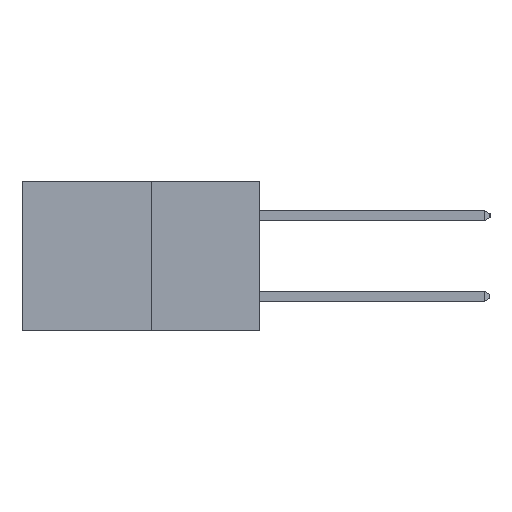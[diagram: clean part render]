
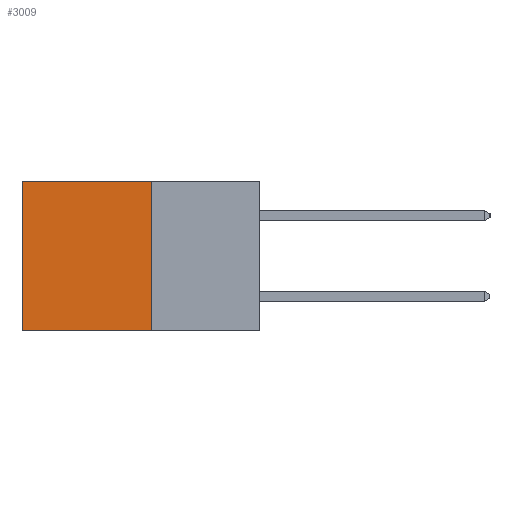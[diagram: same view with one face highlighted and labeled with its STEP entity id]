
A CAD part, left-side view. The second image highlights one B-rep face of the part: STEP entity #3009.
In plain terms, the highlighted planar face has unit normal (-1, 0, 0).
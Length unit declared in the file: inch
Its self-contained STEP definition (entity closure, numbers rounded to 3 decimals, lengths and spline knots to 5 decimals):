
#1442 = CARTESIAN_POINT ( 'NONE',  ( 0.277, 0.27, 0. ) ) ;
#1507 = DIRECTION ( 'NONE',  ( 0., 0., -1. ) ) ;
#1745 = CARTESIAN_POINT ( 'NONE',  ( 0.277, 0.59, -0.37 ) ) ;
#1864 = LINE ( 'NONE', #1745, #9454 ) ;
#1906 = ORIENTED_EDGE ( 'NONE', *, *, #1978, .F. ) ;
#1978 = EDGE_CURVE ( 'NONE', #2466, #4831, #8914, .T. ) ;
#2058 = AXIS2_PLACEMENT_3D ( 'NONE', #5462, #4256, #4336 ) ;
#2251 = EDGE_LOOP ( 'NONE', ( #9683, #1906, #9900, #2403 ) ) ;
#2360 = DIRECTION ( 'NONE',  ( 0., 1., 0. ) ) ;
#2403 = ORIENTED_EDGE ( 'NONE', *, *, #3739, .T. ) ;
#2466 = VERTEX_POINT ( 'NONE', #8448 ) ;
#3009 = ADVANCED_FACE ( 'NONE', ( #5293 ), #5412, .F. ) ;
#3052 = LINE ( 'NONE', #9658, #6705 ) ;
#3739 = EDGE_CURVE ( 'NONE', #8622, #4681, #6283, .T. ) ;
#4256 = DIRECTION ( 'NONE',  ( 1., 0., 0. ) ) ;
#4336 = DIRECTION ( 'NONE',  ( 0., 0., -1. ) ) ;
#4681 = VERTEX_POINT ( 'NONE', #7333 ) ;
#4831 = VERTEX_POINT ( 'NONE', #5152 ) ;
#5152 = CARTESIAN_POINT ( 'NONE',  ( 0.277, 0.59, -0.37 ) ) ;
#5293 = FACE_OUTER_BOUND ( 'NONE', #2251, .T. ) ;
#5303 = CARTESIAN_POINT ( 'NONE',  ( 0.277, 0.27, -0.37 ) ) ;
#5412 = PLANE ( 'NONE',  #2058 ) ;
#5462 = CARTESIAN_POINT ( 'NONE',  ( 0.277, 0.27, -0.37 ) ) ;
#6283 = LINE ( 'NONE', #9169, #9410 ) ;
#6705 = VECTOR ( 'NONE', #9589, 39.37008 ) ;
#7333 = CARTESIAN_POINT ( 'NONE',  ( 0.277, 0.59, 0. ) ) ;
#8153 = EDGE_CURVE ( 'NONE', #4681, #4831, #1864, .T. ) ;
#8427 = VECTOR ( 'NONE', #9919, 39.37008 ) ;
#8448 = CARTESIAN_POINT ( 'NONE',  ( 0.277, 0.27, -0.37 ) ) ;
#8622 = VERTEX_POINT ( 'NONE', #1442 ) ;
#8914 = LINE ( 'NONE', #5303, #8427 ) ;
#9169 = CARTESIAN_POINT ( 'NONE',  ( 0.277, 0.27, 0. ) ) ;
#9217 = EDGE_CURVE ( 'NONE', #8622, #2466, #3052, .T. ) ;
#9410 = VECTOR ( 'NONE', #2360, 39.37008 ) ;
#9454 = VECTOR ( 'NONE', #1507, 39.37008 ) ;
#9589 = DIRECTION ( 'NONE',  ( 0., 0., -1. ) ) ;
#9658 = CARTESIAN_POINT ( 'NONE',  ( 0.277, 0.27, -0.37 ) ) ;
#9683 = ORIENTED_EDGE ( 'NONE', *, *, #8153, .T. ) ;
#9900 = ORIENTED_EDGE ( 'NONE', *, *, #9217, .F. ) ;
#9919 = DIRECTION ( 'NONE',  ( 0., 1., 0. ) ) ;
